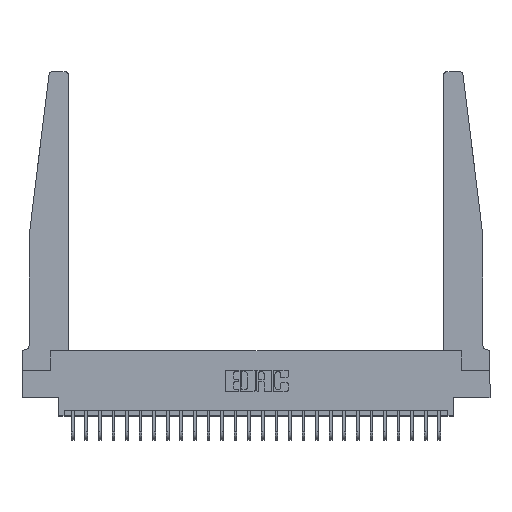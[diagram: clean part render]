
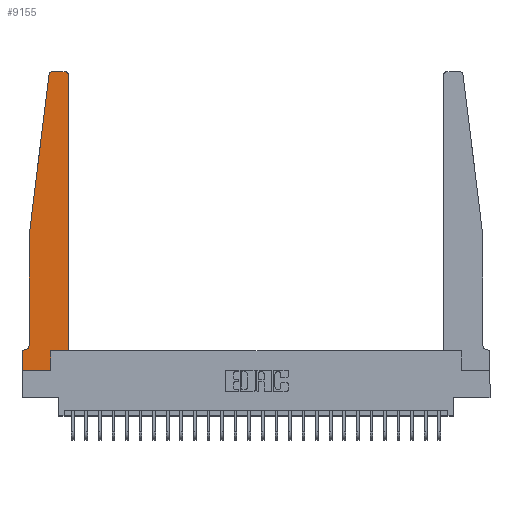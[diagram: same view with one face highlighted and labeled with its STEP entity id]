
A CAD part, top view. The second image highlights one B-rep face of the part: STEP entity #9155.
In plain terms, the highlighted planar face has unit normal (0, 0, 1).
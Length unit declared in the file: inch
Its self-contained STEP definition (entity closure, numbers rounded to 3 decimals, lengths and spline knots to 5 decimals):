
#277 = CARTESIAN_POINT ( 'NONE',  ( 0.015, 0.2375, 0.37 ) ) ;
#356 = CARTESIAN_POINT ( 'NONE',  ( 0.2605, 0.18, 0.37 ) ) ;
#1421 = VECTOR ( 'NONE', #19023, 39.37008 ) ;
#1742 = CARTESIAN_POINT ( 'NONE',  ( 0.2605, 0., 0.37 ) ) ;
#1976 = CARTESIAN_POINT ( 'NONE',  ( 0.065, 1.25, 0.37 ) ) ;
#2769 = VERTEX_POINT ( 'NONE', #17293 ) ;
#2813 = DIRECTION ( 'NONE',  ( 1., 0., 0. ) ) ;
#2884 = VECTOR ( 'NONE', #5666, 39.37008 ) ;
#2996 = LINE ( 'NONE', #14633, #17637 ) ;
#3819 = AXIS2_PLACEMENT_3D ( 'NONE', #9973, #22128, #9877 ) ;
#3913 = CARTESIAN_POINT ( 'NONE',  ( 0.425, 0.18, 0.37 ) ) ;
#3916 = VECTOR ( 'NONE', #23479, 39.37008 ) ;
#4320 = ORIENTED_EDGE ( 'NONE', *, *, #9185, .T. ) ;
#4390 = VERTEX_POINT ( 'NONE', #3913 ) ;
#4401 = ORIENTED_EDGE ( 'NONE', *, *, #18971, .T. ) ;
#4494 = CIRCLE ( 'NONE', #3819, 0.03 ) ;
#4505 = CARTESIAN_POINT ( 'NONE',  ( 0.25, 2.75, 0.37 ) ) ;
#4530 = CARTESIAN_POINT ( 'NONE',  ( 0.015, 0.1875, 0.37 ) ) ;
#4766 = EDGE_CURVE ( 'NONE', #2769, #6337, #4494, .T. ) ;
#5128 = EDGE_CURVE ( 'NONE', #6511, #21217, #14164, .T. ) ;
#5165 = ORIENTED_EDGE ( 'NONE', *, *, #8944, .T. ) ;
#5239 = CARTESIAN_POINT ( 'NONE',  ( 0.065, 0.1875, 0.37 ) ) ;
#5552 = ORIENTED_EDGE ( 'NONE', *, *, #21483, .T. ) ;
#5600 = CARTESIAN_POINT ( 'NONE',  ( 0.425, 0.18, 0.37 ) ) ;
#5666 = DIRECTION ( 'NONE',  ( 0., -1., 0. ) ) ;
#6018 = ORIENTED_EDGE ( 'NONE', *, *, #18724, .T. ) ;
#6292 = CARTESIAN_POINT ( 'NONE',  ( 0., 0., 0.37 ) ) ;
#6337 = VERTEX_POINT ( 'NONE', #18993 ) ;
#6430 = AXIS2_PLACEMENT_3D ( 'NONE', #277, #23052, #6488 ) ;
#6488 = DIRECTION ( 'NONE',  ( -1., 0., 0. ) ) ;
#6511 = VERTEX_POINT ( 'NONE', #6865 ) ;
#6706 = ORIENTED_EDGE ( 'NONE', *, *, #5128, .T. ) ;
#6865 = CARTESIAN_POINT ( 'NONE',  ( 0.065, 0.2375, 0.37 ) ) ;
#7370 = EDGE_CURVE ( 'NONE', #4390, #7531, #26407, .T. ) ;
#7531 = VERTEX_POINT ( 'NONE', #13023 ) ;
#7609 = LINE ( 'NONE', #356, #1421 ) ;
#8337 = CARTESIAN_POINT ( 'NONE',  ( 0., 0.1875, 0.37 ) ) ;
#8944 = EDGE_CURVE ( 'NONE', #6337, #17750, #14329, .T. ) ;
#9155 = ADVANCED_FACE ( 'NONE', ( #9424 ), #19513, .T. ) ;
#9185 = EDGE_CURVE ( 'NONE', #7531, #13838, #22506, .T. ) ;
#9272 = DIRECTION ( 'NONE',  ( 1., 0., 0. ) ) ;
#9359 = EDGE_LOOP ( 'NONE', ( #26522, #12976, #5165, #17952, #6706, #5552, #22533, #19348, #6018, #4401, #21220, #4320 ) ) ;
#9393 = VERTEX_POINT ( 'NONE', #6292 ) ;
#9424 = FACE_OUTER_BOUND ( 'NONE', #9359, .T. ) ;
#9877 = DIRECTION ( 'NONE',  ( 1., 0., 0. ) ) ;
#9973 = CARTESIAN_POINT ( 'NONE',  ( 0.27653, 2.72, 0.37 ) ) ;
#10153 = VERTEX_POINT ( 'NONE', #19849 ) ;
#10269 = LINE ( 'NONE', #25203, #11534 ) ;
#10321 = EDGE_CURVE ( 'NONE', #26258, #9393, #22119, .T. ) ;
#10620 = CARTESIAN_POINT ( 'NONE',  ( 0.395, 2.72, 0.37 ) ) ;
#11038 = DIRECTION ( 'NONE',  ( 1., 0., 0. ) ) ;
#11362 = LINE ( 'NONE', #5239, #18895 ) ;
#11534 = VECTOR ( 'NONE', #22977, 39.37008 ) ;
#12361 = VECTOR ( 'NONE', #18406, 39.37008 ) ;
#12586 = DIRECTION ( 'NONE',  ( 0., -1., 0. ) ) ;
#12976 = ORIENTED_EDGE ( 'NONE', *, *, #4766, .T. ) ;
#13023 = CARTESIAN_POINT ( 'NONE',  ( 0.425, 2.72, 0.37 ) ) ;
#13838 = VERTEX_POINT ( 'NONE', #16582 ) ;
#13917 = DIRECTION ( 'NONE',  ( 0., 1., 0. ) ) ;
#14036 = VECTOR ( 'NONE', #13917, 39.37008 ) ;
#14164 = CIRCLE ( 'NONE', #6430, 0.05 ) ;
#14329 = LINE ( 'NONE', #22717, #12361 ) ;
#14633 = CARTESIAN_POINT ( 'NONE',  ( 0.065, 1.25, 0.37 ) ) ;
#15223 = DIRECTION ( 'NONE',  ( 0., 0., 1. ) ) ;
#15592 = EDGE_CURVE ( 'NONE', #13838, #2769, #18515, .T. ) ;
#15602 = CARTESIAN_POINT ( 'NONE',  ( 0., 0.1875, 0.37 ) ) ;
#15631 = AXIS2_PLACEMENT_3D ( 'NONE', #10620, #15223, #2813 ) ;
#16001 = LINE ( 'NONE', #19165, #19966 ) ;
#16582 = CARTESIAN_POINT ( 'NONE',  ( 0.395, 2.75, 0.37 ) ) ;
#17059 = AXIS2_PLACEMENT_3D ( 'NONE', #8337, #24017, #9272 ) ;
#17293 = CARTESIAN_POINT ( 'NONE',  ( 0.27653, 2.75, 0.37 ) ) ;
#17637 = VECTOR ( 'NONE', #12586, 39.37008 ) ;
#17750 = VERTEX_POINT ( 'NONE', #1976 ) ;
#17952 = ORIENTED_EDGE ( 'NONE', *, *, #19879, .T. ) ;
#18406 = DIRECTION ( 'NONE',  ( -0.122, -0.992, 0. ) ) ;
#18515 = LINE ( 'NONE', #4505, #3916 ) ;
#18724 = EDGE_CURVE ( 'NONE', #24418, #10153, #7609, .T. ) ;
#18895 = VECTOR ( 'NONE', #24093, 39.37008 ) ;
#18971 = EDGE_CURVE ( 'NONE', #10153, #4390, #16001, .T. ) ;
#18993 = CARTESIAN_POINT ( 'NONE',  ( 0.24675, 2.72367, 0.37 ) ) ;
#19023 = DIRECTION ( 'NONE',  ( 0., 1., 0. ) ) ;
#19165 = CARTESIAN_POINT ( 'NONE',  ( 0.425, 0.18, 0.37 ) ) ;
#19348 = ORIENTED_EDGE ( 'NONE', *, *, #22070, .T. ) ;
#19513 = PLANE ( 'NONE',  #17059 ) ;
#19849 = CARTESIAN_POINT ( 'NONE',  ( 0.2605, 0.18, 0.37 ) ) ;
#19879 = EDGE_CURVE ( 'NONE', #17750, #6511, #2996, .T. ) ;
#19966 = VECTOR ( 'NONE', #11038, 39.37008 ) ;
#20133 = CARTESIAN_POINT ( 'NONE',  ( 0., 0., 0.37 ) ) ;
#21217 = VERTEX_POINT ( 'NONE', #4530 ) ;
#21220 = ORIENTED_EDGE ( 'NONE', *, *, #7370, .T. ) ;
#21483 = EDGE_CURVE ( 'NONE', #21217, #26258, #11362, .T. ) ;
#22070 = EDGE_CURVE ( 'NONE', #9393, #24418, #10269, .T. ) ;
#22119 = LINE ( 'NONE', #20133, #2884 ) ;
#22128 = DIRECTION ( 'NONE',  ( 0., 0., 1. ) ) ;
#22506 = CIRCLE ( 'NONE', #15631, 0.03 ) ;
#22533 = ORIENTED_EDGE ( 'NONE', *, *, #10321, .T. ) ;
#22717 = CARTESIAN_POINT ( 'NONE',  ( 0.065, 1.25, 0.37 ) ) ;
#22977 = DIRECTION ( 'NONE',  ( 1., 0., 0. ) ) ;
#23052 = DIRECTION ( 'NONE',  ( 0., 0., -1. ) ) ;
#23479 = DIRECTION ( 'NONE',  ( -1., 0., 0. ) ) ;
#24017 = DIRECTION ( 'NONE',  ( 0., 0., 1. ) ) ;
#24093 = DIRECTION ( 'NONE',  ( -1., 0., 0. ) ) ;
#24418 = VERTEX_POINT ( 'NONE', #1742 ) ;
#25203 = CARTESIAN_POINT ( 'NONE',  ( 0., 0., 0.37 ) ) ;
#26258 = VERTEX_POINT ( 'NONE', #15602 ) ;
#26407 = LINE ( 'NONE', #5600, #14036 ) ;
#26522 = ORIENTED_EDGE ( 'NONE', *, *, #15592, .T. ) ;
